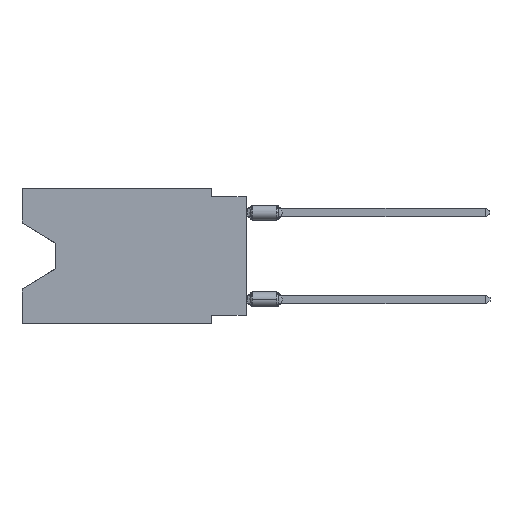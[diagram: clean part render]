
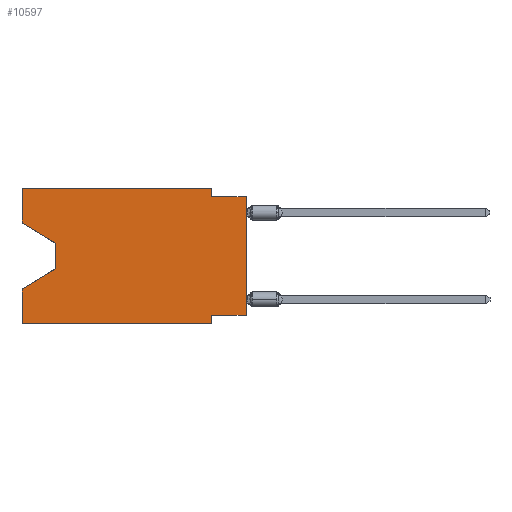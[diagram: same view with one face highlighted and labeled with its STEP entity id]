
A CAD part, left-side view. The second image highlights one B-rep face of the part: STEP entity #10597.
In plain terms, the highlighted planar face has unit normal (-1, 0, 0).
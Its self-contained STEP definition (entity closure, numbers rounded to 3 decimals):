
#132 = CARTESIAN_POINT ( 'NONE',  ( 0., 2.54, -9.271 ) ) ;
#287 = VECTOR ( 'NONE', #11588, 1000. ) ;
#496 = VECTOR ( 'NONE', #21483, 1000. ) ;
#887 = VERTEX_POINT ( 'NONE', #22608 ) ;
#1621 = EDGE_CURVE ( 'NONE', #21168, #23524, #15316, .T. ) ;
#2152 = FACE_OUTER_BOUND ( 'NONE', #18800, .T. ) ;
#2402 = LINE ( 'NONE', #7540, #25543 ) ;
#2846 = DIRECTION ( 'NONE',  ( 0., -1., 0. ) ) ;
#3353 = LINE ( 'NONE', #23989, #21892 ) ;
#3417 = CARTESIAN_POINT ( 'NONE',  ( 0., 13.97, -5.893 ) ) ;
#3696 = CARTESIAN_POINT ( 'NONE',  ( 0., 13.97, -5.893 ) ) ;
#3798 = CARTESIAN_POINT ( 'NONE',  ( 0., 2.54, -9.906 ) ) ;
#4344 = CARTESIAN_POINT ( 'NONE',  ( 0., 16.383, 0. ) ) ;
#4416 = EDGE_CURVE ( 'NONE', #25535, #24266, #13771, .T. ) ;
#4869 = ORIENTED_EDGE ( 'NONE', *, *, #1621, .T. ) ;
#4946 = CARTESIAN_POINT ( 'NONE',  ( 0., 16.383, 0. ) ) ;
#5195 = CARTESIAN_POINT ( 'NONE',  ( 0., 2.54, -0.635 ) ) ;
#5323 = CARTESIAN_POINT ( 'NONE',  ( 0., 0., 0. ) ) ;
#5330 = VERTEX_POINT ( 'NONE', #12179 ) ;
#5467 = ORIENTED_EDGE ( 'NONE', *, *, #10943, .T. ) ;
#5852 = ORIENTED_EDGE ( 'NONE', *, *, #10338, .F. ) ;
#6085 = PLANE ( 'NONE',  #11797 ) ;
#6265 = DIRECTION ( 'NONE',  ( 0., -1., 0. ) ) ;
#6857 = ORIENTED_EDGE ( 'NONE', *, *, #18138, .F. ) ;
#7540 = CARTESIAN_POINT ( 'NONE',  ( 0., 16.383, 0. ) ) ;
#7619 = LINE ( 'NONE', #5323, #11248 ) ;
#7953 = VECTOR ( 'NONE', #18648, 1000. ) ;
#8167 = ORIENTED_EDGE ( 'NONE', *, *, #18786, .F. ) ;
#8400 = ORIENTED_EDGE ( 'NONE', *, *, #4416, .F. ) ;
#8401 = DIRECTION ( 'NONE',  ( 0., 0.855, -0.519 ) ) ;
#8903 = VERTEX_POINT ( 'NONE', #27306 ) ;
#9234 = VERTEX_POINT ( 'NONE', #20743 ) ;
#9240 = CARTESIAN_POINT ( 'NONE',  ( 0., 16.383, -2.546 ) ) ;
#9536 = VECTOR ( 'NONE', #8401, 1000. ) ;
#9559 = VECTOR ( 'NONE', #6265, 1000. ) ;
#10338 = EDGE_CURVE ( 'NONE', #26051, #9234, #20459, .T. ) ;
#10597 = ADVANCED_FACE ( 'NONE', ( #2152 ), #6085, .F. ) ;
#10943 = EDGE_CURVE ( 'NONE', #887, #17432, #3353, .T. ) ;
#10944 = CARTESIAN_POINT ( 'NONE',  ( 0., 0., -9.271 ) ) ;
#11248 = VECTOR ( 'NONE', #16924, 1000. ) ;
#11397 = ORIENTED_EDGE ( 'NONE', *, *, #19119, .T. ) ;
#11588 = DIRECTION ( 'NONE',  ( 0., 0., 1. ) ) ;
#11797 = AXIS2_PLACEMENT_3D ( 'NONE', #22791, #29453, #15430 ) ;
#11815 = ORIENTED_EDGE ( 'NONE', *, *, #21061, .F. ) ;
#12051 = VERTEX_POINT ( 'NONE', #5195 ) ;
#12179 = CARTESIAN_POINT ( 'NONE',  ( 0., 13.97, -4.013 ) ) ;
#12208 = ORIENTED_EDGE ( 'NONE', *, *, #19425, .F. ) ;
#12300 = CARTESIAN_POINT ( 'NONE',  ( 0., 2.54, -9.906 ) ) ;
#12462 = CARTESIAN_POINT ( 'NONE',  ( 0., 0., -0.635 ) ) ;
#12668 = DIRECTION ( 'NONE',  ( 0., -0.855, -0.519 ) ) ;
#13622 = CARTESIAN_POINT ( 'NONE',  ( 0., 0., -9.271 ) ) ;
#13771 = LINE ( 'NONE', #13622, #22818 ) ;
#14480 = DIRECTION ( 'NONE',  ( 0., 0., -1. ) ) ;
#14559 = LINE ( 'NONE', #12300, #496 ) ;
#14931 = CARTESIAN_POINT ( 'NONE',  ( 0., 16.383, -2.546 ) ) ;
#15316 = LINE ( 'NONE', #3417, #9536 ) ;
#15430 = DIRECTION ( 'NONE',  ( 0., 0., -1. ) ) ;
#16830 = CARTESIAN_POINT ( 'NONE',  ( 0., 2.54, 0. ) ) ;
#16924 = DIRECTION ( 'NONE',  ( 0., 0., 1. ) ) ;
#17309 = VECTOR ( 'NONE', #2846, 1000. ) ;
#17432 = VERTEX_POINT ( 'NONE', #3798 ) ;
#18138 = EDGE_CURVE ( 'NONE', #9234, #8903, #18821, .T. ) ;
#18648 = DIRECTION ( 'NONE',  ( 0., 0., -1. ) ) ;
#18786 = EDGE_CURVE ( 'NONE', #24266, #17432, #14559, .T. ) ;
#18800 = EDGE_LOOP ( 'NONE', ( #11397, #28631, #4869, #12208, #5467, #8167, #8400, #27847, #27949, #11815, #6857, #5852 ) ) ;
#18821 = LINE ( 'NONE', #4946, #17309 ) ;
#18977 = LINE ( 'NONE', #28478, #22915 ) ;
#19119 = EDGE_CURVE ( 'NONE', #26051, #5330, #28942, .T. ) ;
#19425 = EDGE_CURVE ( 'NONE', #887, #23524, #2402, .T. ) ;
#20459 = LINE ( 'NONE', #4344, #287 ) ;
#20743 = CARTESIAN_POINT ( 'NONE',  ( 0., 16.383, 0. ) ) ;
#21061 = EDGE_CURVE ( 'NONE', #8903, #12051, #27685, .T. ) ;
#21168 = VERTEX_POINT ( 'NONE', #3696 ) ;
#21483 = DIRECTION ( 'NONE',  ( 0., 0., -1. ) ) ;
#21725 = DIRECTION ( 'NONE',  ( 0., -1., 0. ) ) ;
#21892 = VECTOR ( 'NONE', #21725, 1000. ) ;
#22529 = CARTESIAN_POINT ( 'NONE',  ( 0., 0., -0.635 ) ) ;
#22608 = CARTESIAN_POINT ( 'NONE',  ( 0., 16.383, -9.906 ) ) ;
#22674 = EDGE_CURVE ( 'NONE', #5330, #21168, #18977, .T. ) ;
#22791 = CARTESIAN_POINT ( 'NONE',  ( 0., 16.383, 0. ) ) ;
#22818 = VECTOR ( 'NONE', #25375, 1000. ) ;
#22915 = VECTOR ( 'NONE', #14480, 1000. ) ;
#23524 = VERTEX_POINT ( 'NONE', #28519 ) ;
#23989 = CARTESIAN_POINT ( 'NONE',  ( 0., 16.383, -9.906 ) ) ;
#24266 = VERTEX_POINT ( 'NONE', #132 ) ;
#24786 = LINE ( 'NONE', #22529, #9559 ) ;
#25375 = DIRECTION ( 'NONE',  ( 0., 1., 0. ) ) ;
#25468 = DIRECTION ( 'NONE',  ( 0., 0., 1. ) ) ;
#25535 = VERTEX_POINT ( 'NONE', #10944 ) ;
#25543 = VECTOR ( 'NONE', #25468, 1000. ) ;
#25825 = EDGE_CURVE ( 'NONE', #25535, #26693, #7619, .T. ) ;
#26051 = VERTEX_POINT ( 'NONE', #9240 ) ;
#26693 = VERTEX_POINT ( 'NONE', #12462 ) ;
#26835 = EDGE_CURVE ( 'NONE', #12051, #26693, #24786, .T. ) ;
#27306 = CARTESIAN_POINT ( 'NONE',  ( 0., 2.54, 0. ) ) ;
#27450 = VECTOR ( 'NONE', #12668, 1000. ) ;
#27685 = LINE ( 'NONE', #16830, #7953 ) ;
#27847 = ORIENTED_EDGE ( 'NONE', *, *, #25825, .T. ) ;
#27949 = ORIENTED_EDGE ( 'NONE', *, *, #26835, .F. ) ;
#28478 = CARTESIAN_POINT ( 'NONE',  ( 0., 13.97, -4.013 ) ) ;
#28519 = CARTESIAN_POINT ( 'NONE',  ( 0., 16.383, -7.36 ) ) ;
#28631 = ORIENTED_EDGE ( 'NONE', *, *, #22674, .T. ) ;
#28942 = LINE ( 'NONE', #14931, #27450 ) ;
#29453 = DIRECTION ( 'NONE',  ( 1., 0., 0. ) ) ;
